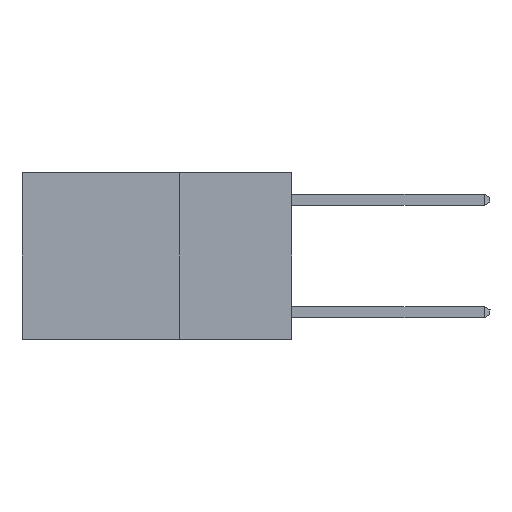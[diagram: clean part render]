
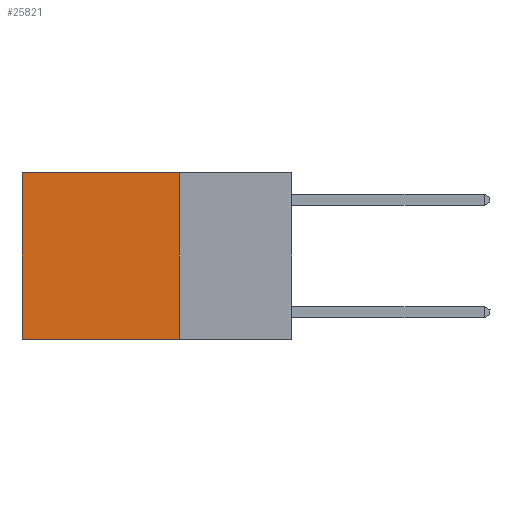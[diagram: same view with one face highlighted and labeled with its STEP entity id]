
A CAD part, left-side view. The second image highlights one B-rep face of the part: STEP entity #25821.
In plain terms, the highlighted planar face has unit normal (-1, 0, 0).
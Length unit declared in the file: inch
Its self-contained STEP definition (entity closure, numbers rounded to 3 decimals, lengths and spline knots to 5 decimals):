
#1313 = LINE ( 'NONE', #10553, #12630 ) ;
#1865 = FACE_OUTER_BOUND ( 'NONE', #11323, .T. ) ;
#2880 = DIRECTION ( 'NONE',  ( 0., 0., -1. ) ) ;
#2910 = ORIENTED_EDGE ( 'NONE', *, *, #21164, .T. ) ;
#2952 = ORIENTED_EDGE ( 'NONE', *, *, #19453, .F. ) ;
#3384 = VERTEX_POINT ( 'NONE', #22450 ) ;
#5118 = CARTESIAN_POINT ( 'NONE',  ( 0.2625, 0.25, 0. ) ) ;
#7087 = VERTEX_POINT ( 'NONE', #27566 ) ;
#7854 = DIRECTION ( 'NONE',  ( 0., 0., -1. ) ) ;
#9130 = LINE ( 'NONE', #19965, #20358 ) ;
#9236 = VECTOR ( 'NONE', #7854, 39.37008 ) ;
#9483 = ORIENTED_EDGE ( 'NONE', *, *, #23067, .T. ) ;
#9496 = CARTESIAN_POINT ( 'NONE',  ( 0.2625, 0.25, 0. ) ) ;
#10120 = AXIS2_PLACEMENT_3D ( 'NONE', #14108, #16346, #2880 ) ;
#10553 = CARTESIAN_POINT ( 'NONE',  ( 0.2625, 0.6, 0. ) ) ;
#11323 = EDGE_LOOP ( 'NONE', ( #2910, #26674, #2952, #9483 ) ) ;
#12630 = VECTOR ( 'NONE', #21710, 39.37008 ) ;
#13939 = VERTEX_POINT ( 'NONE', #9496 ) ;
#14108 = CARTESIAN_POINT ( 'NONE',  ( 0.2625, 0.25, 0. ) ) ;
#15011 = LINE ( 'NONE', #5118, #26228 ) ;
#16346 = DIRECTION ( 'NONE',  ( 1., 0., 0. ) ) ;
#16741 = CARTESIAN_POINT ( 'NONE',  ( 0.2625, 0.25, 0. ) ) ;
#18817 = VERTEX_POINT ( 'NONE', #28078 ) ;
#19453 = EDGE_CURVE ( 'NONE', #13939, #3384, #27058, .T. ) ;
#19965 = CARTESIAN_POINT ( 'NONE',  ( 0.2625, 0.25, -0.37 ) ) ;
#20358 = VECTOR ( 'NONE', #22187, 39.37008 ) ;
#21164 = EDGE_CURVE ( 'NONE', #18817, #7087, #1313, .T. ) ;
#21281 = EDGE_CURVE ( 'NONE', #3384, #7087, #9130, .T. ) ;
#21710 = DIRECTION ( 'NONE',  ( 0., 0., -1. ) ) ;
#22187 = DIRECTION ( 'NONE',  ( 0., 1., 0. ) ) ;
#22450 = CARTESIAN_POINT ( 'NONE',  ( 0.2625, 0.25, -0.37 ) ) ;
#22974 = DIRECTION ( 'NONE',  ( 0., 1., 0. ) ) ;
#23067 = EDGE_CURVE ( 'NONE', #13939, #18817, #15011, .T. ) ;
#25821 = ADVANCED_FACE ( 'NONE', ( #1865 ), #27491, .F. ) ;
#26228 = VECTOR ( 'NONE', #22974, 39.37008 ) ;
#26674 = ORIENTED_EDGE ( 'NONE', *, *, #21281, .F. ) ;
#27058 = LINE ( 'NONE', #16741, #9236 ) ;
#27491 = PLANE ( 'NONE',  #10120 ) ;
#27566 = CARTESIAN_POINT ( 'NONE',  ( 0.2625, 0.6, -0.37 ) ) ;
#28078 = CARTESIAN_POINT ( 'NONE',  ( 0.2625, 0.6, 0. ) ) ;
